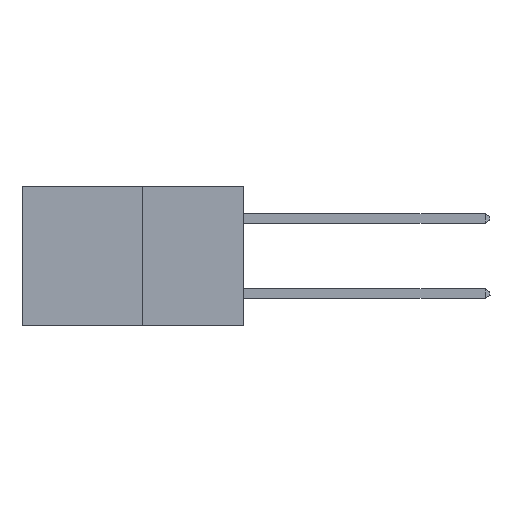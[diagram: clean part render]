
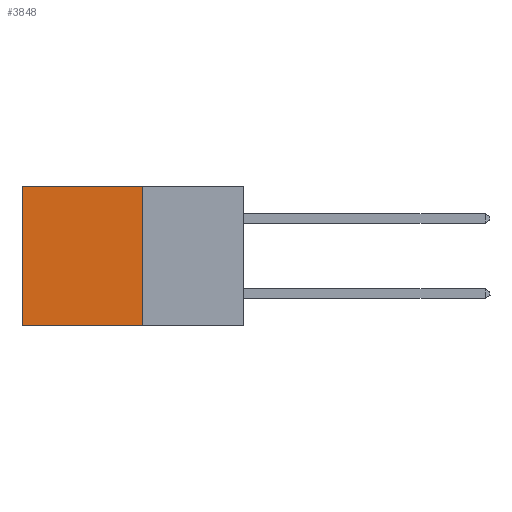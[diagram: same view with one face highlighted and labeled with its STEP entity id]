
A CAD part, left-side view. The second image highlights one B-rep face of the part: STEP entity #3848.
In plain terms, the highlighted planar face has unit normal (-1, 0, 0).
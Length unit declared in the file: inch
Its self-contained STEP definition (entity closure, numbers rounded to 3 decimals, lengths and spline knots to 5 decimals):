
#747 = VERTEX_POINT ( 'NONE', #10316 ) ;
#779 = EDGE_CURVE ( 'NONE', #14351, #747, #12075, .T. ) ;
#1523 = VERTEX_POINT ( 'NONE', #2807 ) ;
#1590 = CARTESIAN_POINT ( 'NONE',  ( 0.277, 0.27, 0. ) ) ;
#1844 = ORIENTED_EDGE ( 'NONE', *, *, #13387, .T. ) ;
#1880 = VECTOR ( 'NONE', #16100, 39.37008 ) ;
#2807 = CARTESIAN_POINT ( 'NONE',  ( 0.277, 0.59, 0. ) ) ;
#3567 = EDGE_LOOP ( 'NONE', ( #1844, #12658, #8240, #12811 ) ) ;
#3709 = VECTOR ( 'NONE', #18968, 39.37008 ) ;
#3848 = ADVANCED_FACE ( 'NONE', ( #16393 ), #4898, .F. ) ;
#3895 = DIRECTION ( 'NONE',  ( 0., 0., -1. ) ) ;
#4118 = VECTOR ( 'NONE', #3895, 39.37008 ) ;
#4164 = LINE ( 'NONE', #14541, #3709 ) ;
#4898 = PLANE ( 'NONE',  #8354 ) ;
#5483 = LINE ( 'NONE', #7218, #16451 ) ;
#6545 = VERTEX_POINT ( 'NONE', #15656 ) ;
#7218 = CARTESIAN_POINT ( 'NONE',  ( 0.277, 0.59, -0.37 ) ) ;
#8240 = ORIENTED_EDGE ( 'NONE', *, *, #779, .F. ) ;
#8354 = AXIS2_PLACEMENT_3D ( 'NONE', #10161, #8572, #15940 ) ;
#8572 = DIRECTION ( 'NONE',  ( 1., 0., 0. ) ) ;
#10161 = CARTESIAN_POINT ( 'NONE',  ( 0.277, 0.27, -0.37 ) ) ;
#10316 = CARTESIAN_POINT ( 'NONE',  ( 0.277, 0.27, -0.37 ) ) ;
#11562 = CARTESIAN_POINT ( 'NONE',  ( 0.277, 0.27, -0.37 ) ) ;
#12075 = LINE ( 'NONE', #11562, #4118 ) ;
#12630 = EDGE_CURVE ( 'NONE', #14351, #1523, #13883, .T. ) ;
#12658 = ORIENTED_EDGE ( 'NONE', *, *, #17710, .F. ) ;
#12811 = ORIENTED_EDGE ( 'NONE', *, *, #12630, .T. ) ;
#13387 = EDGE_CURVE ( 'NONE', #1523, #6545, #5483, .T. ) ;
#13883 = LINE ( 'NONE', #16050, #1880 ) ;
#14351 = VERTEX_POINT ( 'NONE', #1590 ) ;
#14541 = CARTESIAN_POINT ( 'NONE',  ( 0.277, 0.27, -0.37 ) ) ;
#15656 = CARTESIAN_POINT ( 'NONE',  ( 0.277, 0.59, -0.37 ) ) ;
#15940 = DIRECTION ( 'NONE',  ( 0., 0., -1. ) ) ;
#16050 = CARTESIAN_POINT ( 'NONE',  ( 0.277, 0.27, 0. ) ) ;
#16100 = DIRECTION ( 'NONE',  ( 0., 1., 0. ) ) ;
#16393 = FACE_OUTER_BOUND ( 'NONE', #3567, .T. ) ;
#16451 = VECTOR ( 'NONE', #19007, 39.37008 ) ;
#17710 = EDGE_CURVE ( 'NONE', #747, #6545, #4164, .T. ) ;
#18968 = DIRECTION ( 'NONE',  ( 0., 1., 0. ) ) ;
#19007 = DIRECTION ( 'NONE',  ( 0., 0., -1. ) ) ;
